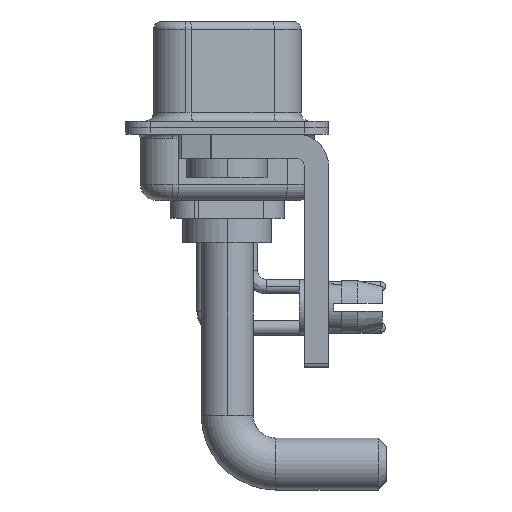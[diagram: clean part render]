
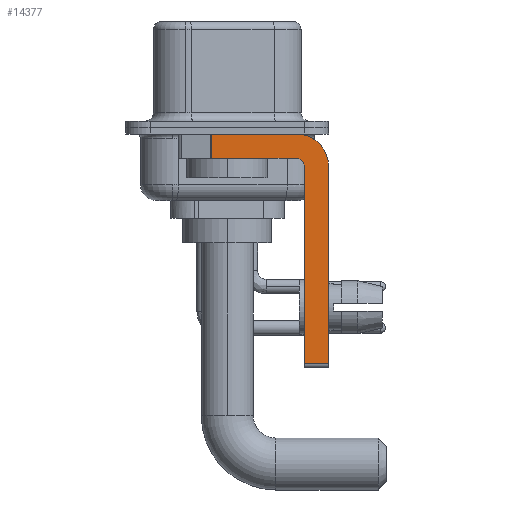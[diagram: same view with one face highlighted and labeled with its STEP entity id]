
A CAD part, left-side view. The second image highlights one B-rep face of the part: STEP entity #14377.
In plain terms, the highlighted planar face has unit normal (-1, 0, 0).
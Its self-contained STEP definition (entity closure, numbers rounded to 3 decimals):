
#52 = CIRCLE ( 'NONE', #19630, 2. ) ;
#425 = CARTESIAN_POINT ( 'NONE',  ( -2.9, -4.75, -14.8 ) ) ;
#1338 = CARTESIAN_POINT ( 'NONE',  ( -2.9, 3., -0.4 ) ) ;
#1452 = VECTOR ( 'NONE', #19724, 1000. ) ;
#2673 = EDGE_CURVE ( 'NONE', #8060, #3403, #10059, .T. ) ;
#2785 = FACE_OUTER_BOUND ( 'NONE', #4711, .T. ) ;
#3282 = CARTESIAN_POINT ( 'NONE',  ( -2.9, 0.978, -1.9 ) ) ;
#3403 = VERTEX_POINT ( 'NONE', #3282 ) ;
#4693 = CIRCLE ( 'NONE', #13316, 0.5 ) ;
#4711 = EDGE_LOOP ( 'NONE', ( #28033, #16797, #20221, #7941, #7709, #10807, #8085, #23267 ) ) ;
#4990 = EDGE_CURVE ( 'NONE', #21313, #5471, #23594, .T. ) ;
#5471 = VERTEX_POINT ( 'NONE', #23040 ) ;
#5747 = DIRECTION ( 'NONE',  ( 0., -1., 0. ) ) ;
#7159 = EDGE_CURVE ( 'NONE', #15888, #5471, #9309, .T. ) ;
#7326 = DIRECTION ( 'NONE',  ( 1., 0., 0. ) ) ;
#7709 = ORIENTED_EDGE ( 'NONE', *, *, #23846, .F. ) ;
#7941 = ORIENTED_EDGE ( 'NONE', *, *, #14573, .F. ) ;
#8023 = LINE ( 'NONE', #1338, #13540 ) ;
#8060 = VERTEX_POINT ( 'NONE', #9106 ) ;
#8085 = ORIENTED_EDGE ( 'NONE', *, *, #4990, .F. ) ;
#8429 = CARTESIAN_POINT ( 'NONE',  ( -2.9, -4.25, -2.4 ) ) ;
#8819 = LINE ( 'NONE', #425, #13180 ) ;
#9106 = CARTESIAN_POINT ( 'NONE',  ( -2.9, 0.978, -0.4 ) ) ;
#9309 = LINE ( 'NONE', #18173, #16275 ) ;
#10059 = LINE ( 'NONE', #12209, #26548 ) ;
#10807 = ORIENTED_EDGE ( 'NONE', *, *, #7159, .T. ) ;
#11055 = CARTESIAN_POINT ( 'NONE',  ( -2.9, -6.25, -2.4 ) ) ;
#11162 = VECTOR ( 'NONE', #19313, 1000. ) ;
#12209 = CARTESIAN_POINT ( 'NONE',  ( -2.9, 0.978, -1.9 ) ) ;
#12314 = EDGE_CURVE ( 'NONE', #8060, #20536, #8023, .T. ) ;
#12455 = CARTESIAN_POINT ( 'NONE',  ( -2.9, -6.25, -2.4 ) ) ;
#12505 = VERTEX_POINT ( 'NONE', #23975 ) ;
#12852 = EDGE_CURVE ( 'NONE', #20536, #21313, #52, .T. ) ;
#13180 = VECTOR ( 'NONE', #15250, 1000. ) ;
#13316 = AXIS2_PLACEMENT_3D ( 'NONE', #8429, #17133, #18466 ) ;
#13321 = EDGE_CURVE ( 'NONE', #12505, #3403, #19214, .T. ) ;
#13540 = VECTOR ( 'NONE', #5747, 1000. ) ;
#14377 = ADVANCED_FACE ( 'NONE', ( #2785 ), #26880, .F. ) ;
#14573 = EDGE_CURVE ( 'NONE', #17593, #12505, #4693, .T. ) ;
#14639 = CARTESIAN_POINT ( 'NONE',  ( -2.9, -4.25, -1.9 ) ) ;
#15250 = DIRECTION ( 'NONE',  ( 0., 0., 1. ) ) ;
#15585 = DIRECTION ( 'NONE',  ( 0., -1., 0. ) ) ;
#15888 = VERTEX_POINT ( 'NONE', #21462 ) ;
#16011 = DIRECTION ( 'NONE',  ( 0., 0., -1. ) ) ;
#16275 = VECTOR ( 'NONE', #15585, 1000. ) ;
#16403 = DIRECTION ( 'NONE',  ( 0., 0., -1. ) ) ;
#16797 = ORIENTED_EDGE ( 'NONE', *, *, #2673, .T. ) ;
#17133 = DIRECTION ( 'NONE',  ( -1., 0., 0. ) ) ;
#17593 = VERTEX_POINT ( 'NONE', #25359 ) ;
#18173 = CARTESIAN_POINT ( 'NONE',  ( -2.9, -4.25, -14.55 ) ) ;
#18466 = DIRECTION ( 'NONE',  ( 0., 0., 1. ) ) ;
#19197 = DIRECTION ( 'NONE',  ( 0., 0., -1. ) ) ;
#19214 = LINE ( 'NONE', #14639, #1452 ) ;
#19313 = DIRECTION ( 'NONE',  ( 0., 0., -1. ) ) ;
#19630 = AXIS2_PLACEMENT_3D ( 'NONE', #20975, #27261, #16403 ) ;
#19724 = DIRECTION ( 'NONE',  ( 0., 1., 0. ) ) ;
#20221 = ORIENTED_EDGE ( 'NONE', *, *, #13321, .F. ) ;
#20314 = CARTESIAN_POINT ( 'NONE',  ( -2.9, -4.25, -2.4 ) ) ;
#20536 = VERTEX_POINT ( 'NONE', #23042 ) ;
#20975 = CARTESIAN_POINT ( 'NONE',  ( -2.9, -4.25, -2.4 ) ) ;
#21313 = VERTEX_POINT ( 'NONE', #11055 ) ;
#21462 = CARTESIAN_POINT ( 'NONE',  ( -2.9, -4.75, -14.55 ) ) ;
#23040 = CARTESIAN_POINT ( 'NONE',  ( -2.9, -6.25, -14.55 ) ) ;
#23042 = CARTESIAN_POINT ( 'NONE',  ( -2.9, -4.25, -0.4 ) ) ;
#23267 = ORIENTED_EDGE ( 'NONE', *, *, #12852, .F. ) ;
#23594 = LINE ( 'NONE', #12455, #11162 ) ;
#23846 = EDGE_CURVE ( 'NONE', #15888, #17593, #8819, .T. ) ;
#23975 = CARTESIAN_POINT ( 'NONE',  ( -2.9, -4.25, -1.9 ) ) ;
#25359 = CARTESIAN_POINT ( 'NONE',  ( -2.9, -4.75, -2.4 ) ) ;
#26548 = VECTOR ( 'NONE', #19197, 1000. ) ;
#26880 = PLANE ( 'NONE',  #27472 ) ;
#27261 = DIRECTION ( 'NONE',  ( 1., 0., 0. ) ) ;
#27472 = AXIS2_PLACEMENT_3D ( 'NONE', #20314, #7326, #16011 ) ;
#28033 = ORIENTED_EDGE ( 'NONE', *, *, #12314, .F. ) ;
